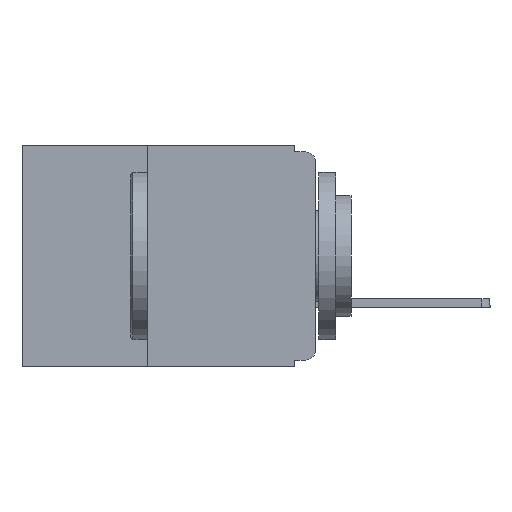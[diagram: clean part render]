
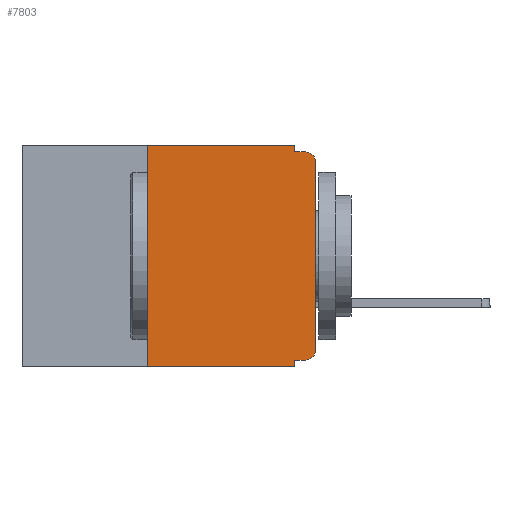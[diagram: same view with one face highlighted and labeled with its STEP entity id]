
A CAD part, left-side view. The second image highlights one B-rep face of the part: STEP entity #7803.
In plain terms, the highlighted planar face has unit normal (-1, 0, 0).
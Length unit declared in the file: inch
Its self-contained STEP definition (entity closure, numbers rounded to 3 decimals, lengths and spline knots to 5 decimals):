
#112 = ORIENTED_EDGE ( 'NONE', *, *, #15776, .F. ) ;
#489 = ORIENTED_EDGE ( 'NONE', *, *, #25479, .F. ) ;
#588 = DIRECTION ( 'NONE',  ( 0., -1., 0. ) ) ;
#609 = FACE_OUTER_BOUND ( 'NONE', #27188, .T. ) ;
#994 = LINE ( 'NONE', #14917, #6213 ) ;
#1283 = LINE ( 'NONE', #16588, #5788 ) ;
#1569 = VERTEX_POINT ( 'NONE', #25721 ) ;
#1910 = EDGE_CURVE ( 'NONE', #19052, #1569, #15135, .T. ) ;
#2169 = CARTESIAN_POINT ( 'NONE',  ( 0., 0.015, -0.32 ) ) ;
#2415 = VERTEX_POINT ( 'NONE', #3636 ) ;
#2684 = AXIS2_PLACEMENT_3D ( 'NONE', #7199, #22658, #9501 ) ;
#3115 = DIRECTION ( 'NONE',  ( 0., 0., 1. ) ) ;
#3216 = DIRECTION ( 'NONE',  ( 0., 0., -1. ) ) ;
#3220 = DIRECTION ( 'NONE',  ( 1., 0., 0. ) ) ;
#3636 = CARTESIAN_POINT ( 'NONE',  ( 0., 0.25, -0.33 ) ) ;
#4235 = VERTEX_POINT ( 'NONE', #10072 ) ;
#4638 = ORIENTED_EDGE ( 'NONE', *, *, #13517, .T. ) ;
#4827 = VECTOR ( 'NONE', #18932, 39.37008 ) ;
#5461 = CARTESIAN_POINT ( 'NONE',  ( 0., 0.015, -0.025 ) ) ;
#5788 = VECTOR ( 'NONE', #23271, 39.37008 ) ;
#6213 = VECTOR ( 'NONE', #8409, 39.37008 ) ;
#6643 = VECTOR ( 'NONE', #3216, 39.37008 ) ;
#7129 = CARTESIAN_POINT ( 'NONE',  ( 0., 0.25, 0. ) ) ;
#7199 = CARTESIAN_POINT ( 'NONE',  ( 0., 0.015, -0.305 ) ) ;
#7244 = EDGE_CURVE ( 'NONE', #2415, #25099, #10789, .T. ) ;
#7323 = CARTESIAN_POINT ( 'NONE',  ( 0., 0.031, -0.33 ) ) ;
#7730 = DIRECTION ( 'NONE',  ( 0., 0., -1. ) ) ;
#7803 = ADVANCED_FACE ( 'NONE', ( #609 ), #9790, .F. ) ;
#8409 = DIRECTION ( 'NONE',  ( 0., 0., 1. ) ) ;
#9006 = EDGE_CURVE ( 'NONE', #9053, #19052, #1283, .T. ) ;
#9053 = VERTEX_POINT ( 'NONE', #12367 ) ;
#9350 = VECTOR ( 'NONE', #588, 39.37008 ) ;
#9501 = DIRECTION ( 'NONE',  ( 0., 0., -1. ) ) ;
#9778 = CARTESIAN_POINT ( 'NONE',  ( 0., 0.25, -0.33 ) ) ;
#9790 = PLANE ( 'NONE',  #23484 ) ;
#10072 = CARTESIAN_POINT ( 'NONE',  ( 0., 0., -0.305 ) ) ;
#10789 = LINE ( 'NONE', #14460, #4827 ) ;
#11897 = CIRCLE ( 'NONE', #13454, 0.015 ) ;
#11960 = ORIENTED_EDGE ( 'NONE', *, *, #21855, .T. ) ;
#12055 = CARTESIAN_POINT ( 'NONE',  ( 0., 0.031, -0.33 ) ) ;
#12367 = CARTESIAN_POINT ( 'NONE',  ( 0., 0.031, 0. ) ) ;
#12999 = DIRECTION ( 'NONE',  ( 0., -1., 0. ) ) ;
#13081 = CARTESIAN_POINT ( 'NONE',  ( 0., 0.031, -0.32 ) ) ;
#13288 = ORIENTED_EDGE ( 'NONE', *, *, #1910, .F. ) ;
#13454 = AXIS2_PLACEMENT_3D ( 'NONE', #5461, #20948, #7730 ) ;
#13517 = EDGE_CURVE ( 'NONE', #4235, #16920, #994, .T. ) ;
#14102 = LINE ( 'NONE', #21793, #19304 ) ;
#14460 = CARTESIAN_POINT ( 'NONE',  ( 0., 0.437, -0.33 ) ) ;
#14917 = CARTESIAN_POINT ( 'NONE',  ( 0., 0., 0. ) ) ;
#15053 = ORIENTED_EDGE ( 'NONE', *, *, #15636, .T. ) ;
#15135 = LINE ( 'NONE', #20302, #9350 ) ;
#15372 = ORIENTED_EDGE ( 'NONE', *, *, #9006, .F. ) ;
#15636 = EDGE_CURVE ( 'NONE', #26712, #4235, #15985, .T. ) ;
#15776 = EDGE_CURVE ( 'NONE', #22158, #25099, #19122, .T. ) ;
#15972 = VERTEX_POINT ( 'NONE', #7129 ) ;
#15985 = CIRCLE ( 'NONE', #2684, 0.015 ) ;
#16588 = CARTESIAN_POINT ( 'NONE',  ( 0., 0.031, 0. ) ) ;
#16920 = VERTEX_POINT ( 'NONE', #19550 ) ;
#17456 = ORIENTED_EDGE ( 'NONE', *, *, #18117, .F. ) ;
#18117 = EDGE_CURVE ( 'NONE', #15972, #9053, #14102, .T. ) ;
#18709 = DIRECTION ( 'NONE',  ( 0., 0., -1. ) ) ;
#18872 = ORIENTED_EDGE ( 'NONE', *, *, #28310, .F. ) ;
#18932 = DIRECTION ( 'NONE',  ( 0., -1., 0. ) ) ;
#19052 = VERTEX_POINT ( 'NONE', #24155 ) ;
#19122 = LINE ( 'NONE', #12055, #6643 ) ;
#19304 = VECTOR ( 'NONE', #12999, 39.37008 ) ;
#19550 = CARTESIAN_POINT ( 'NONE',  ( 0., 0., -0.025 ) ) ;
#19915 = VECTOR ( 'NONE', #28429, 39.37008 ) ;
#20302 = CARTESIAN_POINT ( 'NONE',  ( 0., 0., -0.01 ) ) ;
#20806 = VECTOR ( 'NONE', #3115, 39.37008 ) ;
#20948 = DIRECTION ( 'NONE',  ( -1., 0., 0. ) ) ;
#21793 = CARTESIAN_POINT ( 'NONE',  ( 0., 0.437, 0. ) ) ;
#21855 = EDGE_CURVE ( 'NONE', #16920, #1569, #11897, .T. ) ;
#22158 = VERTEX_POINT ( 'NONE', #13081 ) ;
#22658 = DIRECTION ( 'NONE',  ( -1., 0., 0. ) ) ;
#23271 = DIRECTION ( 'NONE',  ( 0., 0., -1. ) ) ;
#23484 = AXIS2_PLACEMENT_3D ( 'NONE', #25258, #3220, #18709 ) ;
#24155 = CARTESIAN_POINT ( 'NONE',  ( 0., 0.031, -0.01 ) ) ;
#25097 = LINE ( 'NONE', #26268, #19915 ) ;
#25099 = VERTEX_POINT ( 'NONE', #7323 ) ;
#25258 = CARTESIAN_POINT ( 'NONE',  ( 0., 0.437, 0. ) ) ;
#25479 = EDGE_CURVE ( 'NONE', #26712, #22158, #25097, .T. ) ;
#25721 = CARTESIAN_POINT ( 'NONE',  ( 0., 0.015, -0.01 ) ) ;
#26268 = CARTESIAN_POINT ( 'NONE',  ( 0., 0., -0.32 ) ) ;
#26597 = LINE ( 'NONE', #9778, #20806 ) ;
#26712 = VERTEX_POINT ( 'NONE', #2169 ) ;
#26738 = ORIENTED_EDGE ( 'NONE', *, *, #7244, .T. ) ;
#27188 = EDGE_LOOP ( 'NONE', ( #4638, #11960, #13288, #15372, #17456, #18872, #26738, #112, #489, #15053 ) ) ;
#28310 = EDGE_CURVE ( 'NONE', #2415, #15972, #26597, .T. ) ;
#28429 = DIRECTION ( 'NONE',  ( 0., 1., 0. ) ) ;
